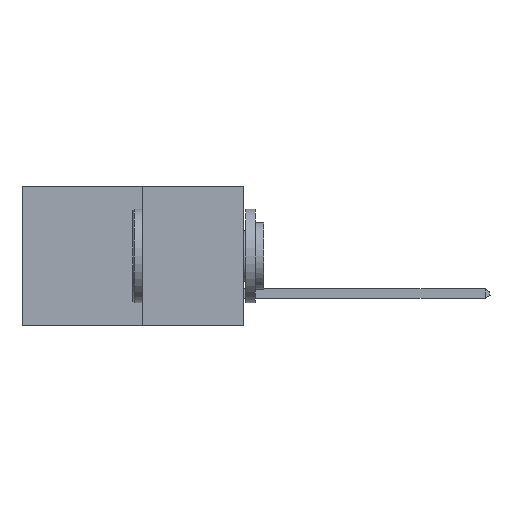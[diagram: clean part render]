
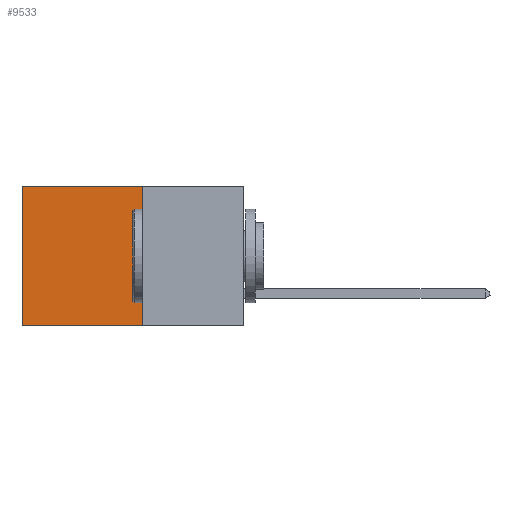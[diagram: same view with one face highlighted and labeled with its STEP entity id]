
A CAD part, left-side view. The second image highlights one B-rep face of the part: STEP entity #9533.
In plain terms, the highlighted planar face has unit normal (-1, 0, 0).
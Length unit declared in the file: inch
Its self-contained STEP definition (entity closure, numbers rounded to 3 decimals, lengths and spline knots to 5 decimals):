
#367 = CARTESIAN_POINT ( 'NONE',  ( 0.277, 0.59, -0.37 ) ) ;
#459 = DIRECTION ( 'NONE',  ( 0., 0., -1. ) ) ;
#554 = PLANE ( 'NONE',  #7254 ) ;
#1507 = VECTOR ( 'NONE', #11607, 39.37008 ) ;
#1823 = DIRECTION ( 'NONE',  ( 0., 0., -1. ) ) ;
#2407 = EDGE_LOOP ( 'NONE', ( #4849, #9565, #7585, #9081 ) ) ;
#2424 = LINE ( 'NONE', #367, #11411 ) ;
#2707 = VERTEX_POINT ( 'NONE', #3991 ) ;
#2750 = VERTEX_POINT ( 'NONE', #5548 ) ;
#3008 = CARTESIAN_POINT ( 'NONE',  ( 0.277, 0.59, 0. ) ) ;
#3083 = VERTEX_POINT ( 'NONE', #3008 ) ;
#3991 = CARTESIAN_POINT ( 'NONE',  ( 0.277, 0.27, -0.37 ) ) ;
#4849 = ORIENTED_EDGE ( 'NONE', *, *, #4956, .T. ) ;
#4859 = DIRECTION ( 'NONE',  ( 0., 0., -1. ) ) ;
#4956 = EDGE_CURVE ( 'NONE', #3083, #10089, #2424, .T. ) ;
#5193 = VECTOR ( 'NONE', #13354, 39.37008 ) ;
#5548 = CARTESIAN_POINT ( 'NONE',  ( 0.277, 0.27, 0. ) ) ;
#5748 = EDGE_CURVE ( 'NONE', #2707, #10089, #11350, .T. ) ;
#7254 = AXIS2_PLACEMENT_3D ( 'NONE', #14543, #9046, #1823 ) ;
#7585 = ORIENTED_EDGE ( 'NONE', *, *, #11013, .F. ) ;
#7961 = EDGE_CURVE ( 'NONE', #2750, #3083, #11284, .T. ) ;
#9046 = DIRECTION ( 'NONE',  ( 1., 0., 0. ) ) ;
#9081 = ORIENTED_EDGE ( 'NONE', *, *, #7961, .T. ) ;
#9533 = ADVANCED_FACE ( 'NONE', ( #13159 ), #554, .F. ) ;
#9565 = ORIENTED_EDGE ( 'NONE', *, *, #5748, .F. ) ;
#10089 = VERTEX_POINT ( 'NONE', #14354 ) ;
#11013 = EDGE_CURVE ( 'NONE', #2750, #2707, #12768, .T. ) ;
#11284 = LINE ( 'NONE', #12726, #1507 ) ;
#11350 = LINE ( 'NONE', #12259, #5193 ) ;
#11411 = VECTOR ( 'NONE', #459, 39.37008 ) ;
#11607 = DIRECTION ( 'NONE',  ( 0., 1., 0. ) ) ;
#12079 = VECTOR ( 'NONE', #4859, 39.37008 ) ;
#12259 = CARTESIAN_POINT ( 'NONE',  ( 0.277, 0.27, -0.37 ) ) ;
#12726 = CARTESIAN_POINT ( 'NONE',  ( 0.277, 0.27, 0. ) ) ;
#12768 = LINE ( 'NONE', #14900, #12079 ) ;
#13159 = FACE_OUTER_BOUND ( 'NONE', #2407, .T. ) ;
#13354 = DIRECTION ( 'NONE',  ( 0., 1., 0. ) ) ;
#14354 = CARTESIAN_POINT ( 'NONE',  ( 0.277, 0.59, -0.37 ) ) ;
#14543 = CARTESIAN_POINT ( 'NONE',  ( 0.277, 0.27, -0.37 ) ) ;
#14900 = CARTESIAN_POINT ( 'NONE',  ( 0.277, 0.27, -0.37 ) ) ;
